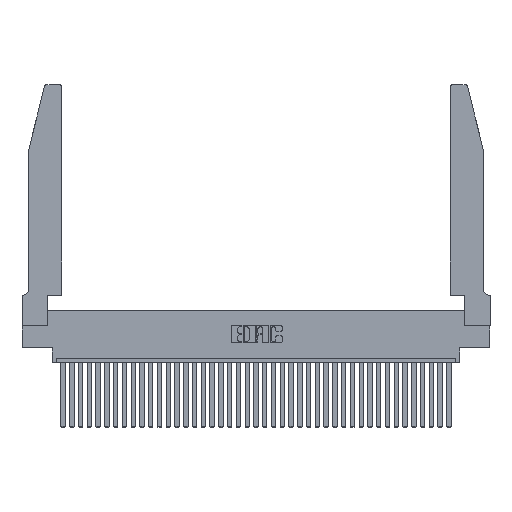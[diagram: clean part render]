
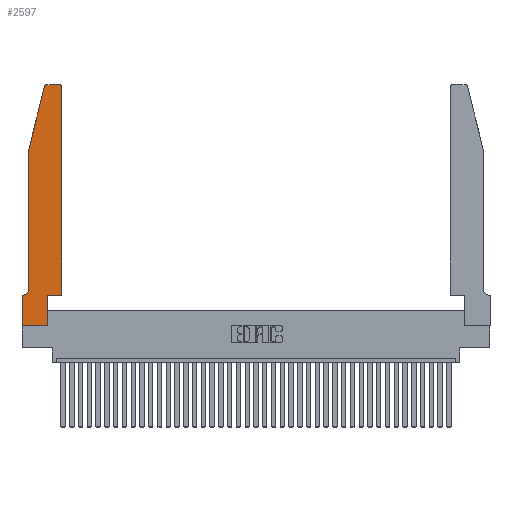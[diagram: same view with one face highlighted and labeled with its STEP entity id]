
A CAD part, top view. The second image highlights one B-rep face of the part: STEP entity #2597.
In plain terms, the highlighted planar face has unit normal (0, 0, 1).
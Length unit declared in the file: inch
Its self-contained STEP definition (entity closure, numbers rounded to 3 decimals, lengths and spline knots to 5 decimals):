
#260 = DIRECTION ( 'NONE',  ( -1., 0., 0. ) ) ;
#834 = VECTOR ( 'NONE', #36304, 39.37008 ) ;
#840 = CARTESIAN_POINT ( 'NONE',  ( 0.0055, 0.42, 0.37 ) ) ;
#857 = DIRECTION ( 'NONE',  ( 0., 0., 1. ) ) ;
#974 = EDGE_CURVE ( 'NONE', #2305, #10678, #24720, .T. ) ;
#1199 = LINE ( 'NONE', #7923, #24819 ) ;
#1500 = VECTOR ( 'NONE', #36938, 39.37008 ) ;
#1691 = ORIENTED_EDGE ( 'NONE', *, *, #23443, .T. ) ;
#1867 = AXIS2_PLACEMENT_3D ( 'NONE', #18588, #24540, #18723 ) ;
#2305 = VERTEX_POINT ( 'NONE', #26504 ) ;
#2347 = CARTESIAN_POINT ( 'NONE',  ( 0.0755, 2., 0.37 ) ) ;
#2597 = ADVANCED_FACE ( 'NONE', ( #20001 ), #32675, .T. ) ;
#2747 = LINE ( 'NONE', #19219, #27186 ) ;
#2783 = VECTOR ( 'NONE', #17674, 39.37008 ) ;
#3212 = VERTEX_POINT ( 'NONE', #13386 ) ;
#3778 = DIRECTION ( 'NONE',  ( 0., 0., 1. ) ) ;
#4085 = CARTESIAN_POINT ( 'NONE',  ( 0.4205, 2.72, 0.37 ) ) ;
#4192 = DIRECTION ( 'NONE',  ( -1., 0., 0. ) ) ;
#5366 = VECTOR ( 'NONE', #25505, 39.37008 ) ;
#5535 = CARTESIAN_POINT ( 'NONE',  ( 0.284, 2.75, 0.37 ) ) ;
#5686 = ORIENTED_EDGE ( 'NONE', *, *, #12612, .T. ) ;
#6494 = CARTESIAN_POINT ( 'NONE',  ( 0.284, 2.72, 0.37 ) ) ;
#6662 = ORIENTED_EDGE ( 'NONE', *, *, #974, .T. ) ;
#6927 = EDGE_CURVE ( 'NONE', #10678, #23596, #2747, .T. ) ;
#7525 = DIRECTION ( 'NONE',  ( 0., 1., 0. ) ) ;
#7923 = CARTESIAN_POINT ( 'NONE',  ( 0.2865, 0.35, 0.37 ) ) ;
#10027 = CARTESIAN_POINT ( 'NONE',  ( 0., 0., 0.37 ) ) ;
#10372 = EDGE_CURVE ( 'NONE', #3212, #23766, #11230, .T. ) ;
#10678 = VERTEX_POINT ( 'NONE', #2347 ) ;
#11230 = LINE ( 'NONE', #30792, #1500 ) ;
#12136 = CARTESIAN_POINT ( 'NONE',  ( 0., 0.35, 0.37 ) ) ;
#12545 = LINE ( 'NONE', #16141, #32414 ) ;
#12548 = VERTEX_POINT ( 'NONE', #22733 ) ;
#12612 = EDGE_CURVE ( 'NONE', #19965, #27744, #23581, .T. ) ;
#12684 = CARTESIAN_POINT ( 'NONE',  ( 0.2865, 0.35, 0.37 ) ) ;
#12809 = CARTESIAN_POINT ( 'NONE',  ( 0.0755, 2., 0.37 ) ) ;
#13159 = EDGE_LOOP ( 'NONE', ( #26226, #36348, #6662, #29866, #23721, #5686, #17754, #1691, #31426, #24696, #20398, #30515 ) ) ;
#13386 = CARTESIAN_POINT ( 'NONE',  ( 0.4505, 0.35, 0.37 ) ) ;
#13809 = EDGE_CURVE ( 'NONE', #27744, #12548, #28562, .T. ) ;
#14923 = AXIS2_PLACEMENT_3D ( 'NONE', #4085, #857, #33755 ) ;
#16141 = CARTESIAN_POINT ( 'NONE',  ( 0., 0., 0.37 ) ) ;
#16172 = VERTEX_POINT ( 'NONE', #12684 ) ;
#16201 = DIRECTION ( 'NONE',  ( -0.239, -0.971, 0. ) ) ;
#16922 = CARTESIAN_POINT ( 'NONE',  ( 0.4205, 2.75, 0.37 ) ) ;
#17674 = DIRECTION ( 'NONE',  ( -1., 0., 0. ) ) ;
#17703 = CARTESIAN_POINT ( 'NONE',  ( 0.0755, 0.42, 0.37 ) ) ;
#17754 = ORIENTED_EDGE ( 'NONE', *, *, #13809, .T. ) ;
#18338 = AXIS2_PLACEMENT_3D ( 'NONE', #6494, #3778, #33189 ) ;
#18588 = CARTESIAN_POINT ( 'NONE',  ( 0., 0.35, 0.37 ) ) ;
#18723 = DIRECTION ( 'NONE',  ( 1., 0., 0. ) ) ;
#19127 = EDGE_CURVE ( 'NONE', #24544, #2305, #24257, .T. ) ;
#19219 = CARTESIAN_POINT ( 'NONE',  ( 0.0755, 2., 0.37 ) ) ;
#19902 = CARTESIAN_POINT ( 'NONE',  ( 0.0055, 0.35, 0.37 ) ) ;
#19965 = VERTEX_POINT ( 'NONE', #19902 ) ;
#20001 = FACE_OUTER_BOUND ( 'NONE', #13159, .T. ) ;
#20293 = EDGE_CURVE ( 'NONE', #23766, #37117, #33029, .T. ) ;
#20398 = ORIENTED_EDGE ( 'NONE', *, *, #10372, .T. ) ;
#20603 = CARTESIAN_POINT ( 'NONE',  ( 0.2865, 0., 0.37 ) ) ;
#21474 = DIRECTION ( 'NONE',  ( 0., 0., -1. ) ) ;
#22291 = DIRECTION ( 'NONE',  ( 1., 0., 0. ) ) ;
#22733 = CARTESIAN_POINT ( 'NONE',  ( 0., 0., 0.37 ) ) ;
#23443 = EDGE_CURVE ( 'NONE', #12548, #36254, #12545, .T. ) ;
#23581 = LINE ( 'NONE', #32115, #2783 ) ;
#23596 = VERTEX_POINT ( 'NONE', #17703 ) ;
#23721 = ORIENTED_EDGE ( 'NONE', *, *, #26570, .T. ) ;
#23766 = VERTEX_POINT ( 'NONE', #25902 ) ;
#24257 = CIRCLE ( 'NONE', #18338, 0.03 ) ;
#24540 = DIRECTION ( 'NONE',  ( 0., 0., 1. ) ) ;
#24544 = VERTEX_POINT ( 'NONE', #5535 ) ;
#24696 = ORIENTED_EDGE ( 'NONE', *, *, #28402, .T. ) ;
#24720 = LINE ( 'NONE', #12809, #34864 ) ;
#24819 = VECTOR ( 'NONE', #7525, 39.37008 ) ;
#24969 = AXIS2_PLACEMENT_3D ( 'NONE', #840, #21474, #4192 ) ;
#25505 = DIRECTION ( 'NONE',  ( 1., 0., 0. ) ) ;
#25902 = CARTESIAN_POINT ( 'NONE',  ( 0.4505, 2.72, 0.37 ) ) ;
#26226 = ORIENTED_EDGE ( 'NONE', *, *, #37931, .T. ) ;
#26504 = CARTESIAN_POINT ( 'NONE',  ( 0.25487, 2.72718, 0.37 ) ) ;
#26570 = EDGE_CURVE ( 'NONE', #23596, #19965, #34148, .T. ) ;
#26746 = LINE ( 'NONE', #29678, #35029 ) ;
#27186 = VECTOR ( 'NONE', #36834, 39.37008 ) ;
#27744 = VERTEX_POINT ( 'NONE', #12136 ) ;
#28393 = EDGE_CURVE ( 'NONE', #36254, #16172, #1199, .T. ) ;
#28402 = EDGE_CURVE ( 'NONE', #16172, #3212, #29836, .T. ) ;
#28562 = LINE ( 'NONE', #10027, #834 ) ;
#29678 = CARTESIAN_POINT ( 'NONE',  ( 0.2605, 2.75, 0.37 ) ) ;
#29836 = LINE ( 'NONE', #34126, #5366 ) ;
#29866 = ORIENTED_EDGE ( 'NONE', *, *, #6927, .T. ) ;
#30515 = ORIENTED_EDGE ( 'NONE', *, *, #20293, .T. ) ;
#30792 = CARTESIAN_POINT ( 'NONE',  ( 0.4505, 0.35, 0.37 ) ) ;
#31426 = ORIENTED_EDGE ( 'NONE', *, *, #28393, .T. ) ;
#32115 = CARTESIAN_POINT ( 'NONE',  ( 0.0755, 0.35, 0.37 ) ) ;
#32414 = VECTOR ( 'NONE', #22291, 39.37008 ) ;
#32675 = PLANE ( 'NONE',  #1867 ) ;
#33029 = CIRCLE ( 'NONE', #14923, 0.03 ) ;
#33189 = DIRECTION ( 'NONE',  ( 1., 0., 0. ) ) ;
#33755 = DIRECTION ( 'NONE',  ( 1., 0., 0. ) ) ;
#34126 = CARTESIAN_POINT ( 'NONE',  ( 0.4505, 0.35, 0.37 ) ) ;
#34148 = CIRCLE ( 'NONE', #24969, 0.07 ) ;
#34864 = VECTOR ( 'NONE', #16201, 39.37008 ) ;
#35029 = VECTOR ( 'NONE', #260, 39.37008 ) ;
#36254 = VERTEX_POINT ( 'NONE', #20603 ) ;
#36304 = DIRECTION ( 'NONE',  ( 0., -1., 0. ) ) ;
#36348 = ORIENTED_EDGE ( 'NONE', *, *, #19127, .T. ) ;
#36834 = DIRECTION ( 'NONE',  ( 0., -1., 0. ) ) ;
#36938 = DIRECTION ( 'NONE',  ( 0., 1., 0. ) ) ;
#37117 = VERTEX_POINT ( 'NONE', #16922 ) ;
#37931 = EDGE_CURVE ( 'NONE', #37117, #24544, #26746, .T. ) ;
